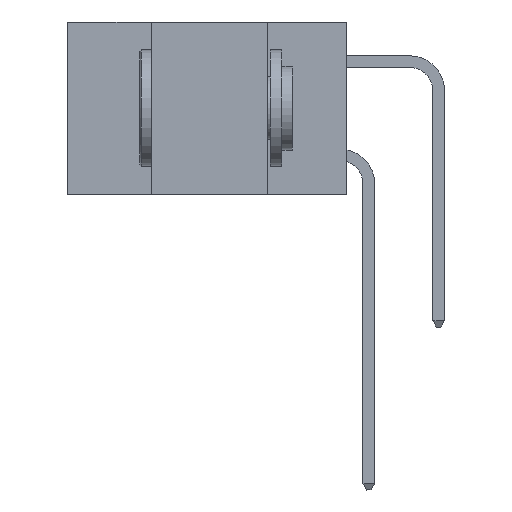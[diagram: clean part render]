
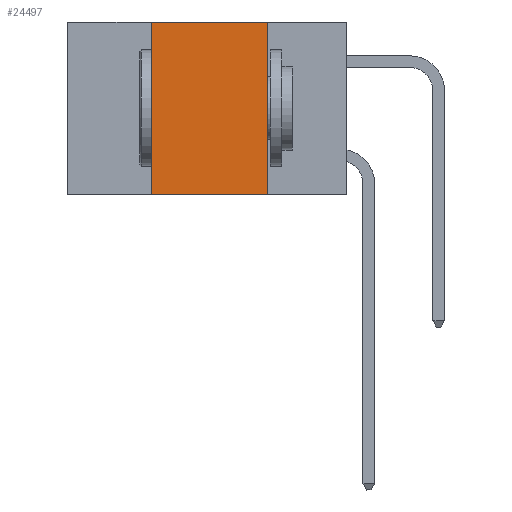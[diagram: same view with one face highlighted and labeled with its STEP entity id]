
A CAD part, left-side view. The second image highlights one B-rep face of the part: STEP entity #24497.
In plain terms, the highlighted planar face has unit normal (-1, 0, 0).
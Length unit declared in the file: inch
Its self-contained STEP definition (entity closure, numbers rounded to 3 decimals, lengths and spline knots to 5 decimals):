
#14 = LINE ( 'NONE', #1696, #32826 ) ;
#581 = DIRECTION ( 'NONE',  ( 0., 0., -1. ) ) ;
#975 = VECTOR ( 'NONE', #20087, 39.37008 ) ;
#1015 = FACE_OUTER_BOUND ( 'NONE', #13739, .T. ) ;
#1088 = CARTESIAN_POINT ( 'NONE',  ( 0., 0.17, 0. ) ) ;
#1561 = ORIENTED_EDGE ( 'NONE', *, *, #12313, .F. ) ;
#1696 = CARTESIAN_POINT ( 'NONE',  ( 0., 0.6, -0.37 ) ) ;
#1807 = EDGE_CURVE ( 'NONE', #16695, #16953, #19341, .T. ) ;
#2394 = PLANE ( 'NONE',  #11667 ) ;
#4648 = ORIENTED_EDGE ( 'NONE', *, *, #1807, .F. ) ;
#5712 = DIRECTION ( 'NONE',  ( 0., -1., 0. ) ) ;
#6405 = EDGE_CURVE ( 'NONE', #17434, #16953, #14, .T. ) ;
#6640 = VECTOR ( 'NONE', #581, 39.37008 ) ;
#9096 = ORIENTED_EDGE ( 'NONE', *, *, #19842, .F. ) ;
#11097 = VECTOR ( 'NONE', #39269, 39.37008 ) ;
#11165 = CARTESIAN_POINT ( 'NONE',  ( 0., 0.6, 0. ) ) ;
#11667 = AXIS2_PLACEMENT_3D ( 'NONE', #29700, #20635, #23439 ) ;
#12313 = EDGE_CURVE ( 'NONE', #17434, #14595, #12525, .T. ) ;
#12525 = LINE ( 'NONE', #24989, #11097 ) ;
#13739 = EDGE_LOOP ( 'NONE', ( #4648, #9096, #1561, #19028 ) ) ;
#14595 = VERTEX_POINT ( 'NONE', #22058 ) ;
#15621 = CARTESIAN_POINT ( 'NONE',  ( 0., 0.42, -0.37 ) ) ;
#16695 = VERTEX_POINT ( 'NONE', #1088 ) ;
#16953 = VERTEX_POINT ( 'NONE', #18579 ) ;
#17434 = VERTEX_POINT ( 'NONE', #15621 ) ;
#18579 = CARTESIAN_POINT ( 'NONE',  ( 0., 0.17, -0.37 ) ) ;
#19028 = ORIENTED_EDGE ( 'NONE', *, *, #6405, .T. ) ;
#19341 = LINE ( 'NONE', #37239, #6640 ) ;
#19842 = EDGE_CURVE ( 'NONE', #14595, #16695, #28086, .T. ) ;
#20087 = DIRECTION ( 'NONE',  ( 0., -1., 0. ) ) ;
#20635 = DIRECTION ( 'NONE',  ( 1., 0., 0. ) ) ;
#22058 = CARTESIAN_POINT ( 'NONE',  ( 0., 0.42, 0. ) ) ;
#23439 = DIRECTION ( 'NONE',  ( 0., 0., -1. ) ) ;
#24497 = ADVANCED_FACE ( 'NONE', ( #1015 ), #2394, .F. ) ;
#24989 = CARTESIAN_POINT ( 'NONE',  ( 0., 0.42, 0. ) ) ;
#28086 = LINE ( 'NONE', #11165, #975 ) ;
#29700 = CARTESIAN_POINT ( 'NONE',  ( 0., 0.6, 0. ) ) ;
#32826 = VECTOR ( 'NONE', #5712, 39.37008 ) ;
#37239 = CARTESIAN_POINT ( 'NONE',  ( 0., 0.17, 0. ) ) ;
#39269 = DIRECTION ( 'NONE',  ( 0., 0., 1. ) ) ;
